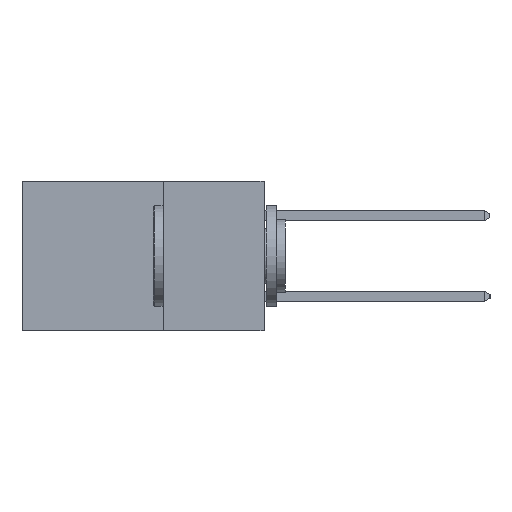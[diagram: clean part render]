
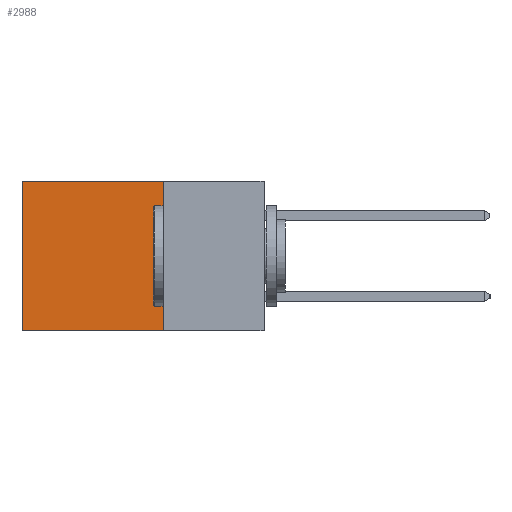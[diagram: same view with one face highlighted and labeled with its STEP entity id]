
A CAD part, left-side view. The second image highlights one B-rep face of the part: STEP entity #2988.
In plain terms, the highlighted planar face has unit normal (-1, 0, 0).
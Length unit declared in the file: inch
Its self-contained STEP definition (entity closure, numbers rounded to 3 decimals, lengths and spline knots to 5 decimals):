
#337 = VERTEX_POINT ( 'NONE', #5245 ) ;
#517 = DIRECTION ( 'NONE',  ( 0., 0., -1. ) ) ;
#726 = DIRECTION ( 'NONE',  ( 1., 0., 0. ) ) ;
#917 = DIRECTION ( 'NONE',  ( 0., 1., 0. ) ) ;
#1582 = VECTOR ( 'NONE', #17770, 39.37008 ) ;
#2988 = ADVANCED_FACE ( 'NONE', ( #15854 ), #10103, .F. ) ;
#3145 = LINE ( 'NONE', #17938, #7308 ) ;
#3270 = EDGE_LOOP ( 'NONE', ( #4817, #16911, #7174, #10810 ) ) ;
#4055 = DIRECTION ( 'NONE',  ( 0., 0., -1. ) ) ;
#4817 = ORIENTED_EDGE ( 'NONE', *, *, #15340, .T. ) ;
#5245 = CARTESIAN_POINT ( 'NONE',  ( 0.2615, 0.6, -0.37 ) ) ;
#5346 = EDGE_CURVE ( 'NONE', #6919, #14124, #3145, .T. ) ;
#5725 = CARTESIAN_POINT ( 'NONE',  ( 0.2615, 0.25, -0.37 ) ) ;
#5730 = VECTOR ( 'NONE', #4055, 39.37008 ) ;
#5786 = LINE ( 'NONE', #11639, #1582 ) ;
#6919 = VERTEX_POINT ( 'NONE', #9144 ) ;
#6932 = CARTESIAN_POINT ( 'NONE',  ( 0.2615, 0.25, -0.37 ) ) ;
#7174 = ORIENTED_EDGE ( 'NONE', *, *, #18169, .F. ) ;
#7308 = VECTOR ( 'NONE', #917, 39.37008 ) ;
#7879 = AXIS2_PLACEMENT_3D ( 'NONE', #6932, #726, #11668 ) ;
#8290 = CARTESIAN_POINT ( 'NONE',  ( 0.2615, 0.6, -0.37 ) ) ;
#9144 = CARTESIAN_POINT ( 'NONE',  ( 0.2615, 0.25, 0. ) ) ;
#9380 = LINE ( 'NONE', #5725, #5730 ) ;
#10103 = PLANE ( 'NONE',  #7879 ) ;
#10783 = VERTEX_POINT ( 'NONE', #12848 ) ;
#10810 = ORIENTED_EDGE ( 'NONE', *, *, #5346, .T. ) ;
#11325 = VECTOR ( 'NONE', #517, 39.37008 ) ;
#11639 = CARTESIAN_POINT ( 'NONE',  ( 0.2615, 0.25, -0.37 ) ) ;
#11668 = DIRECTION ( 'NONE',  ( 0., 0., -1. ) ) ;
#12848 = CARTESIAN_POINT ( 'NONE',  ( 0.2615, 0.25, -0.37 ) ) ;
#14124 = VERTEX_POINT ( 'NONE', #14683 ) ;
#14683 = CARTESIAN_POINT ( 'NONE',  ( 0.2615, 0.6, 0. ) ) ;
#15340 = EDGE_CURVE ( 'NONE', #14124, #337, #15363, .T. ) ;
#15363 = LINE ( 'NONE', #8290, #11325 ) ;
#15854 = FACE_OUTER_BOUND ( 'NONE', #3270, .T. ) ;
#16080 = EDGE_CURVE ( 'NONE', #10783, #337, #5786, .T. ) ;
#16911 = ORIENTED_EDGE ( 'NONE', *, *, #16080, .F. ) ;
#17770 = DIRECTION ( 'NONE',  ( 0., 1., 0. ) ) ;
#17938 = CARTESIAN_POINT ( 'NONE',  ( 0.2615, 0.25, 0. ) ) ;
#18169 = EDGE_CURVE ( 'NONE', #6919, #10783, #9380, .T. ) ;
